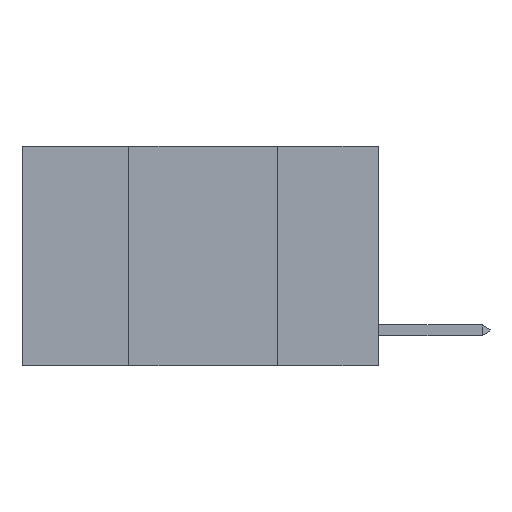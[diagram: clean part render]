
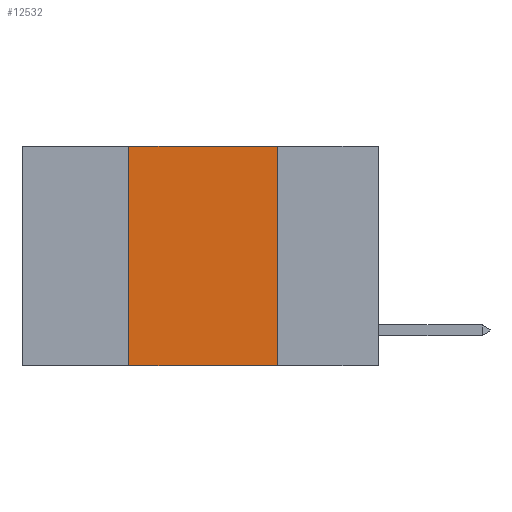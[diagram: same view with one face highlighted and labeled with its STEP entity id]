
A CAD part, left-side view. The second image highlights one B-rep face of the part: STEP entity #12532.
In plain terms, the highlighted planar face has unit normal (-1, 0, 0).
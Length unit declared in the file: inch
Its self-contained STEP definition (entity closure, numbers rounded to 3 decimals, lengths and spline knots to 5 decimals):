
#282 = LINE ( 'NONE', #6788, #6631 ) ;
#498 = LINE ( 'NONE', #24171, #24767 ) ;
#846 = VERTEX_POINT ( 'NONE', #25657 ) ;
#1034 = CARTESIAN_POINT ( 'NONE',  ( 0., 0.42, 0. ) ) ;
#1349 = ORIENTED_EDGE ( 'NONE', *, *, #11601, .F. ) ;
#3476 = FACE_OUTER_BOUND ( 'NONE', #17978, .T. ) ;
#5673 = VECTOR ( 'NONE', #16184, 39.37008 ) ;
#6631 = VECTOR ( 'NONE', #23126, 39.37008 ) ;
#6788 = CARTESIAN_POINT ( 'NONE',  ( 0., 0.42, 0. ) ) ;
#7086 = CARTESIAN_POINT ( 'NONE',  ( 0., 0.6, 0. ) ) ;
#8350 = LINE ( 'NONE', #9305, #26257 ) ;
#9305 = CARTESIAN_POINT ( 'NONE',  ( 0., 0.6, 0. ) ) ;
#10169 = DIRECTION ( 'NONE',  ( 0., 0., -1. ) ) ;
#10445 = DIRECTION ( 'NONE',  ( 0., 0., -1. ) ) ;
#11601 = EDGE_CURVE ( 'NONE', #20873, #27977, #8350, .T. ) ;
#12046 = EDGE_CURVE ( 'NONE', #27977, #22350, #498, .T. ) ;
#12448 = EDGE_CURVE ( 'NONE', #846, #22350, #29826, .T. ) ;
#12532 = ADVANCED_FACE ( 'NONE', ( #3476 ), #28125, .F. ) ;
#13895 = ORIENTED_EDGE ( 'NONE', *, *, #22973, .F. ) ;
#14139 = DIRECTION ( 'NONE',  ( 1., 0., 0. ) ) ;
#16184 = DIRECTION ( 'NONE',  ( 0., -1., 0. ) ) ;
#16234 = DIRECTION ( 'NONE',  ( 0., -1., 0. ) ) ;
#17978 = EDGE_LOOP ( 'NONE', ( #25595, #1349, #13895, #27041 ) ) ;
#18341 = CARTESIAN_POINT ( 'NONE',  ( 0., 0.17, 0. ) ) ;
#20354 = AXIS2_PLACEMENT_3D ( 'NONE', #7086, #14139, #10445 ) ;
#20873 = VERTEX_POINT ( 'NONE', #1034 ) ;
#22350 = VERTEX_POINT ( 'NONE', #22750 ) ;
#22750 = CARTESIAN_POINT ( 'NONE',  ( 0., 0.17, -0.37 ) ) ;
#22973 = EDGE_CURVE ( 'NONE', #846, #20873, #282, .T. ) ;
#23126 = DIRECTION ( 'NONE',  ( 0., 0., 1. ) ) ;
#24171 = CARTESIAN_POINT ( 'NONE',  ( 0., 0.17, 0. ) ) ;
#24767 = VECTOR ( 'NONE', #10169, 39.37008 ) ;
#25595 = ORIENTED_EDGE ( 'NONE', *, *, #12046, .F. ) ;
#25657 = CARTESIAN_POINT ( 'NONE',  ( 0., 0.42, -0.37 ) ) ;
#26257 = VECTOR ( 'NONE', #16234, 39.37008 ) ;
#27041 = ORIENTED_EDGE ( 'NONE', *, *, #12448, .T. ) ;
#27821 = CARTESIAN_POINT ( 'NONE',  ( 0., 0.6, -0.37 ) ) ;
#27977 = VERTEX_POINT ( 'NONE', #18341 ) ;
#28125 = PLANE ( 'NONE',  #20354 ) ;
#29826 = LINE ( 'NONE', #27821, #5673 ) ;
